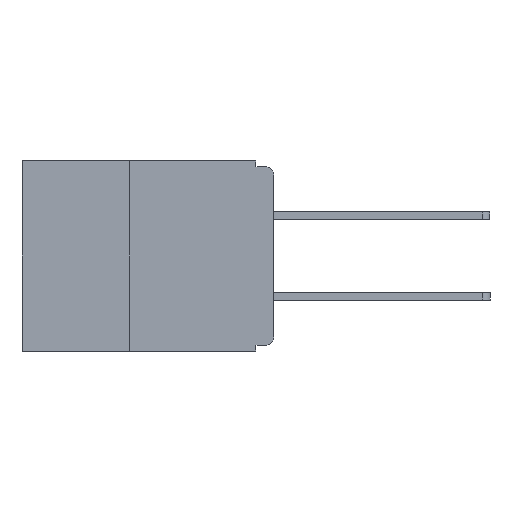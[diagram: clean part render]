
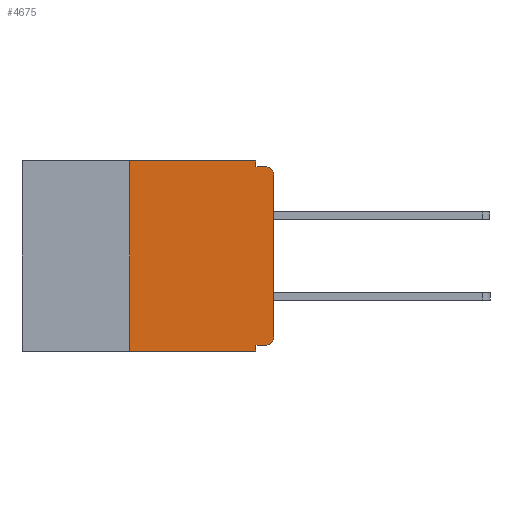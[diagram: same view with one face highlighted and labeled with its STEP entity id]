
A CAD part, left-side view. The second image highlights one B-rep face of the part: STEP entity #4675.
In plain terms, the highlighted planar face has unit normal (-1, 0, 0).
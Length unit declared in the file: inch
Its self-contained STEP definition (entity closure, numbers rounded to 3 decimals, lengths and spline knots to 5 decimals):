
#49 = CARTESIAN_POINT ( 'NONE',  ( 0., 0.031, -0.33 ) ) ;
#105 = ORIENTED_EDGE ( 'NONE', *, *, #14843, .F. ) ;
#268 = CARTESIAN_POINT ( 'NONE',  ( 0., 0.031, 0. ) ) ;
#316 = ORIENTED_EDGE ( 'NONE', *, *, #4549, .F. ) ;
#354 = CARTESIAN_POINT ( 'NONE',  ( 0., 0., -0.305 ) ) ;
#387 = ORIENTED_EDGE ( 'NONE', *, *, #13367, .F. ) ;
#401 = DIRECTION ( 'NONE',  ( 0., -1., 0. ) ) ;
#656 = ORIENTED_EDGE ( 'NONE', *, *, #11084, .T. ) ;
#674 = ORIENTED_EDGE ( 'NONE', *, *, #8806, .F. ) ;
#814 = VECTOR ( 'NONE', #5888, 39.37008 ) ;
#853 = ORIENTED_EDGE ( 'NONE', *, *, #9244, .F. ) ;
#996 = ORIENTED_EDGE ( 'NONE', *, *, #1677, .T. ) ;
#1677 = EDGE_CURVE ( 'NONE', #12214, #13786, #13549, .T. ) ;
#2032 = EDGE_LOOP ( 'NONE', ( #13579, #14250, #14654, #105, #316, #387, #656, #674, #853, #996 ) ) ;
#2073 = DIRECTION ( 'NONE',  ( 0., -1., 0. ) ) ;
#2115 = LINE ( 'NONE', #14878, #14213 ) ;
#2145 = LINE ( 'NONE', #8953, #10896 ) ;
#2401 = VERTEX_POINT ( 'NONE', #12943 ) ;
#3023 = DIRECTION ( 'NONE',  ( 0., 0., 1. ) ) ;
#3808 = VERTEX_POINT ( 'NONE', #6551 ) ;
#4066 = VECTOR ( 'NONE', #3023, 39.37008 ) ;
#4420 = VECTOR ( 'NONE', #2073, 39.37008 ) ;
#4549 = EDGE_CURVE ( 'NONE', #2401, #5959, #8019, .T. ) ;
#4675 = ADVANCED_FACE ( 'NONE', ( #14870 ), #12865, .F. ) ;
#5308 = VERTEX_POINT ( 'NONE', #14789 ) ;
#5888 = DIRECTION ( 'NONE',  ( 0., -1., 0. ) ) ;
#5930 = CARTESIAN_POINT ( 'NONE',  ( 0., 0.031, 0. ) ) ;
#5959 = VERTEX_POINT ( 'NONE', #5930 ) ;
#6200 = LINE ( 'NONE', #268, #14863 ) ;
#6551 = CARTESIAN_POINT ( 'NONE',  ( 0., 0.25, -0.33 ) ) ;
#6556 = LINE ( 'NONE', #8243, #9230 ) ;
#6801 = AXIS2_PLACEMENT_3D ( 'NONE', #12880, #8901, #12270 ) ;
#6986 = DIRECTION ( 'NONE',  ( -1., 0., 0. ) ) ;
#7067 = VERTEX_POINT ( 'NONE', #14421 ) ;
#7339 = LINE ( 'NONE', #10152, #4066 ) ;
#7949 = DIRECTION ( 'NONE',  ( 1., 0., 0. ) ) ;
#8019 = LINE ( 'NONE', #8138, #4420 ) ;
#8118 = CARTESIAN_POINT ( 'NONE',  ( 0., 0.437, 0. ) ) ;
#8138 = CARTESIAN_POINT ( 'NONE',  ( 0., 0.437, 0. ) ) ;
#8243 = CARTESIAN_POINT ( 'NONE',  ( 0., 0., -0.32 ) ) ;
#8270 = DIRECTION ( 'NONE',  ( 0., 1., 0. ) ) ;
#8521 = CARTESIAN_POINT ( 'NONE',  ( 0., 0.031, -0.33 ) ) ;
#8775 = CIRCLE ( 'NONE', #11983, 0.015 ) ;
#8806 = EDGE_CURVE ( 'NONE', #5308, #9212, #12091, .T. ) ;
#8901 = DIRECTION ( 'NONE',  ( -1., 0., 0. ) ) ;
#8953 = CARTESIAN_POINT ( 'NONE',  ( 0., 0., -0.01 ) ) ;
#9011 = DIRECTION ( 'NONE',  ( 0., 0., -1. ) ) ;
#9037 = VECTOR ( 'NONE', #15044, 39.37008 ) ;
#9212 = VERTEX_POINT ( 'NONE', #8521 ) ;
#9230 = VECTOR ( 'NONE', #8270, 39.37008 ) ;
#9244 = EDGE_CURVE ( 'NONE', #12214, #5308, #6556, .T. ) ;
#10152 = CARTESIAN_POINT ( 'NONE',  ( 0., 0., 0. ) ) ;
#10410 = DIRECTION ( 'NONE',  ( 0., 0., 1. ) ) ;
#10896 = VECTOR ( 'NONE', #401, 39.37008 ) ;
#11084 = EDGE_CURVE ( 'NONE', #3808, #9212, #13420, .T. ) ;
#11617 = CARTESIAN_POINT ( 'NONE',  ( 0., 0.437, -0.33 ) ) ;
#11630 = VERTEX_POINT ( 'NONE', #12532 ) ;
#11983 = AXIS2_PLACEMENT_3D ( 'NONE', #13759, #6986, #14872 ) ;
#12091 = LINE ( 'NONE', #49, #9037 ) ;
#12214 = VERTEX_POINT ( 'NONE', #14686 ) ;
#12270 = DIRECTION ( 'NONE',  ( 0., 0., -1. ) ) ;
#12307 = EDGE_CURVE ( 'NONE', #7067, #15091, #8775, .T. ) ;
#12532 = CARTESIAN_POINT ( 'NONE',  ( 0., 0.031, -0.01 ) ) ;
#12591 = EDGE_CURVE ( 'NONE', #11630, #15091, #2145, .T. ) ;
#12865 = PLANE ( 'NONE',  #13740 ) ;
#12880 = CARTESIAN_POINT ( 'NONE',  ( 0., 0.015, -0.305 ) ) ;
#12943 = CARTESIAN_POINT ( 'NONE',  ( 0., 0.25, 0. ) ) ;
#13237 = EDGE_CURVE ( 'NONE', #13786, #7067, #7339, .T. ) ;
#13348 = DIRECTION ( 'NONE',  ( 0., 0., -1. ) ) ;
#13367 = EDGE_CURVE ( 'NONE', #3808, #2401, #2115, .T. ) ;
#13420 = LINE ( 'NONE', #11617, #814 ) ;
#13549 = CIRCLE ( 'NONE', #6801, 0.015 ) ;
#13579 = ORIENTED_EDGE ( 'NONE', *, *, #13237, .T. ) ;
#13740 = AXIS2_PLACEMENT_3D ( 'NONE', #8118, #7949, #9011 ) ;
#13759 = CARTESIAN_POINT ( 'NONE',  ( 0., 0.015, -0.025 ) ) ;
#13786 = VERTEX_POINT ( 'NONE', #354 ) ;
#14213 = VECTOR ( 'NONE', #10410, 39.37008 ) ;
#14250 = ORIENTED_EDGE ( 'NONE', *, *, #12307, .T. ) ;
#14421 = CARTESIAN_POINT ( 'NONE',  ( 0., 0., -0.025 ) ) ;
#14654 = ORIENTED_EDGE ( 'NONE', *, *, #12591, .F. ) ;
#14686 = CARTESIAN_POINT ( 'NONE',  ( 0., 0.015, -0.32 ) ) ;
#14789 = CARTESIAN_POINT ( 'NONE',  ( 0., 0.031, -0.32 ) ) ;
#14843 = EDGE_CURVE ( 'NONE', #5959, #11630, #6200, .T. ) ;
#14863 = VECTOR ( 'NONE', #13348, 39.37008 ) ;
#14870 = FACE_OUTER_BOUND ( 'NONE', #2032, .T. ) ;
#14872 = DIRECTION ( 'NONE',  ( 0., 0., -1. ) ) ;
#14878 = CARTESIAN_POINT ( 'NONE',  ( 0., 0.25, -0.33 ) ) ;
#14929 = CARTESIAN_POINT ( 'NONE',  ( 0., 0.015, -0.01 ) ) ;
#15044 = DIRECTION ( 'NONE',  ( 0., 0., -1. ) ) ;
#15091 = VERTEX_POINT ( 'NONE', #14929 ) ;
